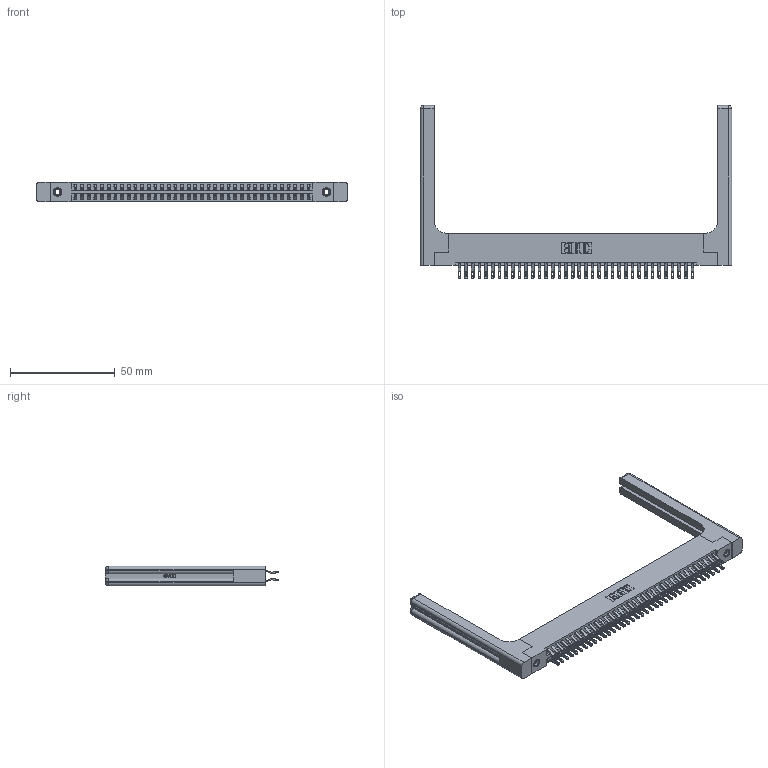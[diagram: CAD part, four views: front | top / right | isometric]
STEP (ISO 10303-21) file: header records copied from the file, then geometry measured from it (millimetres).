
FILE_DESCRIPTION (( 'STEP AP203' ), '1' );
FILE_NAME ('396-072-555-258.STEP', '2019-10-30T20:16:14', ( '' ), ( '' ), 'SwSTEP 2.0', 'SolidWorks 2016', '' );
FILE_SCHEMA (( 'CONFIG_CONTROL_DESIGN' ));
Length unit declared in the file: inch
Products named in the file (5): 396-072-555-258; 345-250-001_345-250-001-102; 346-220-058_345-220-058; 346 Part_Flush Mounting Lugs - 0.156 Dia-TH; 345-292-001_555 Tail
Assembly tree (77 placements, depth 2):
  396-072-555-258
    346 Part_Flush Mounting Lugs - 0.156 Dia-TH
    345-292-001_555 Tail  x72
    345-250-001_345-250-001-102  x2
    346-220-058_345-220-058  x2
Bounding box: 148.36 x 82.42 x 9.4 mm (x, y, z)
Volume: 22123.6 mm3; surface area: 25731.9 mm2
Topology: 77 solids, 77 shells, 4554 faces, 14171 edges, 9426 vertices
Faces by surface type: plane 2600, cylinder 1894, bspline 36, cone 12, sphere 8, torus 4
Entity records: 29810 total; most frequent: CARTESIAN_POINT 5963, ORIENTED_EDGE 4664, DIRECTION 4208, EDGE_CURVE 2332, VECTOR 1944, LINE 1944, VERTEX_POINT 1546, AXIS2_PLACEMENT_3D 1132
